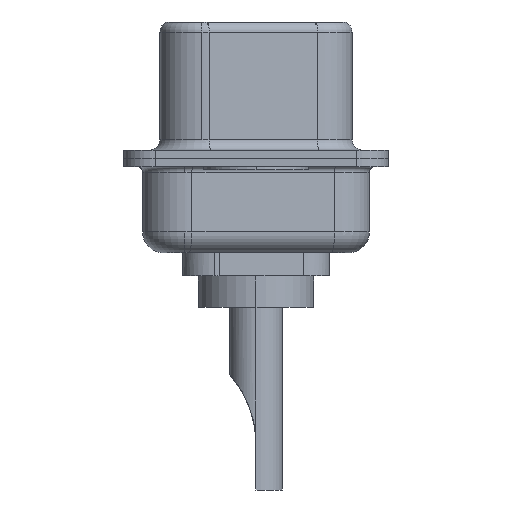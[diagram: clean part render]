
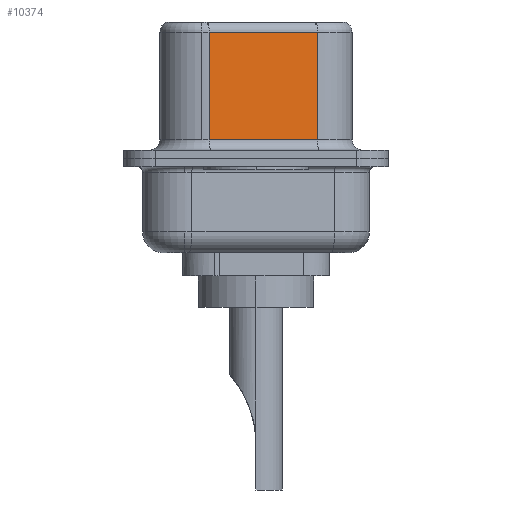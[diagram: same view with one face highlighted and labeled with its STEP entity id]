
A CAD part, left-side view. The second image highlights one B-rep face of the part: STEP entity #10374.
In plain terms, the highlighted planar face has unit normal (-0.985, -0.174, 0).
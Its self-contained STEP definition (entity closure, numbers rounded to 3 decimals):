
#26 = PLANE ( 'NONE',  #9337 ) ;
#224 = VECTOR ( 'NONE', #1978, 1000. ) ;
#230 = EDGE_CURVE ( 'NONE', #3517, #2867, #9519, .T. ) ;
#952 = EDGE_CURVE ( 'NONE', #2867, #3812, #6001, .T. ) ;
#1305 = CARTESIAN_POINT ( 'NONE',  ( 3.67, 2.233, 6.02 ) ) ;
#1487 = VECTOR ( 'NONE', #4745, 1000. ) ;
#1978 = DIRECTION ( 'NONE',  ( 0., 0., -1. ) ) ;
#2729 = ORIENTED_EDGE ( 'NONE', *, *, #10210, .F. ) ;
#2750 = FACE_OUTER_BOUND ( 'NONE', #9456, .T. ) ;
#2867 = VERTEX_POINT ( 'NONE', #1305 ) ;
#2937 = LINE ( 'NONE', #7484, #6636 ) ;
#2953 = DIRECTION ( 'NONE',  ( 0., 0., -1. ) ) ;
#2955 = VERTEX_POINT ( 'NONE', #9120 ) ;
#3517 = VERTEX_POINT ( 'NONE', #12531 ) ;
#3812 = VERTEX_POINT ( 'NONE', #11550 ) ;
#4105 = CARTESIAN_POINT ( 'NONE',  ( 3.67, 2.233, 6.52 ) ) ;
#4339 = ORIENTED_EDGE ( 'NONE', *, *, #952, .T. ) ;
#4399 = CARTESIAN_POINT ( 'NONE',  ( 4.58, -2.927, 6.52 ) ) ;
#4531 = DIRECTION ( 'NONE',  ( -0.174, 0.985, 0. ) ) ;
#4735 = ORIENTED_EDGE ( 'NONE', *, *, #230, .T. ) ;
#4745 = DIRECTION ( 'NONE',  ( 0.174, -0.985, 0. ) ) ;
#6001 = LINE ( 'NONE', #4105, #224 ) ;
#6636 = VECTOR ( 'NONE', #2953, 1000. ) ;
#7484 = CARTESIAN_POINT ( 'NONE',  ( 4.58, -2.927, 6.52 ) ) ;
#8117 = CARTESIAN_POINT ( 'NONE',  ( 4.58, -2.927, 0.9 ) ) ;
#8471 = VECTOR ( 'NONE', #13232, 1000. ) ;
#9120 = CARTESIAN_POINT ( 'NONE',  ( 4.58, -2.927, 0.9 ) ) ;
#9337 = AXIS2_PLACEMENT_3D ( 'NONE', #4399, #12184, #4531 ) ;
#9456 = EDGE_LOOP ( 'NONE', ( #2729, #4735, #4339, #14158 ) ) ;
#9519 = LINE ( 'NONE', #9960, #8471 ) ;
#9960 = CARTESIAN_POINT ( 'NONE',  ( 4.58, -2.927, 6.02 ) ) ;
#10210 = EDGE_CURVE ( 'NONE', #3517, #2955, #2937, .T. ) ;
#10374 = ADVANCED_FACE ( 'NONE', ( #2750 ), #26, .F. ) ;
#11550 = CARTESIAN_POINT ( 'NONE',  ( 3.67, 2.233, 0.9 ) ) ;
#12184 = DIRECTION ( 'NONE',  ( 0.985, 0.174, 0. ) ) ;
#12531 = CARTESIAN_POINT ( 'NONE',  ( 4.58, -2.927, 6.02 ) ) ;
#12896 = EDGE_CURVE ( 'NONE', #3812, #2955, #13633, .T. ) ;
#13232 = DIRECTION ( 'NONE',  ( -0.174, 0.985, 0. ) ) ;
#13633 = LINE ( 'NONE', #8117, #1487 ) ;
#14158 = ORIENTED_EDGE ( 'NONE', *, *, #12896, .T. ) ;
